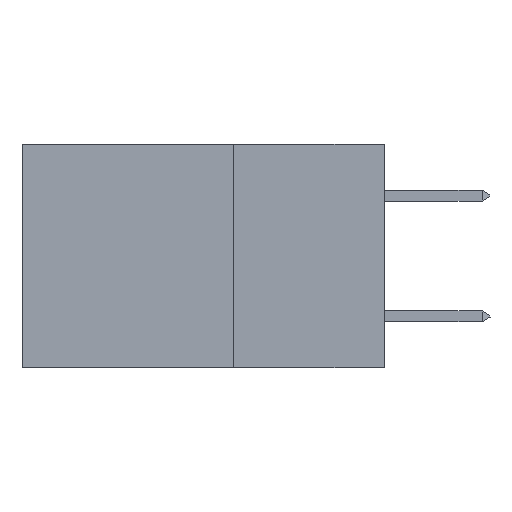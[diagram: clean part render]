
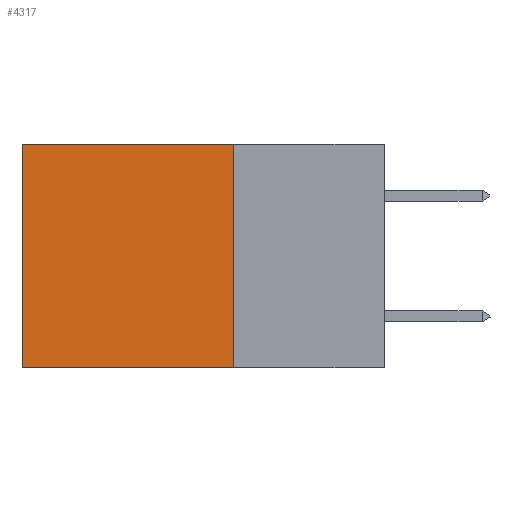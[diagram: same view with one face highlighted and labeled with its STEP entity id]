
A CAD part, left-side view. The second image highlights one B-rep face of the part: STEP entity #4317.
In plain terms, the highlighted planar face has unit normal (-1, 0, 0).
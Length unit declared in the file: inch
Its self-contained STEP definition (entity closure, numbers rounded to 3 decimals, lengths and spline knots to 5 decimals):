
#6 = CARTESIAN_POINT ( 'NONE',  ( 0.2875, 0.25, -0.37 ) ) ;
#36 = ORIENTED_EDGE ( 'NONE', *, *, #13482, .F. ) ;
#254 = ORIENTED_EDGE ( 'NONE', *, *, #1266, .T. ) ;
#265 = EDGE_CURVE ( 'NONE', #1464, #14253, #1152, .T. ) ;
#725 = DIRECTION ( 'NONE',  ( 0., 1., 0. ) ) ;
#787 = VECTOR ( 'NONE', #8856, 39.37008 ) ;
#1096 = DIRECTION ( 'NONE',  ( 0., 1., 0. ) ) ;
#1152 = LINE ( 'NONE', #13448, #787 ) ;
#1266 = EDGE_CURVE ( 'NONE', #7739, #12143, #2345, .T. ) ;
#1464 = VERTEX_POINT ( 'NONE', #4417 ) ;
#1869 = CARTESIAN_POINT ( 'NONE',  ( 0.2875, 0.25, -0.37 ) ) ;
#2345 = LINE ( 'NONE', #13073, #2856 ) ;
#2378 = DIRECTION ( 'NONE',  ( 1., 0., 0. ) ) ;
#2856 = VECTOR ( 'NONE', #13174, 39.37008 ) ;
#2892 = EDGE_CURVE ( 'NONE', #1464, #7739, #4488, .T. ) ;
#3500 = LINE ( 'NONE', #1869, #11552 ) ;
#4007 = ORIENTED_EDGE ( 'NONE', *, *, #2892, .T. ) ;
#4317 = ADVANCED_FACE ( 'NONE', ( #4813 ), #6948, .F. ) ;
#4417 = CARTESIAN_POINT ( 'NONE',  ( 0.2875, 0.25, 0. ) ) ;
#4488 = LINE ( 'NONE', #6894, #11859 ) ;
#4813 = FACE_OUTER_BOUND ( 'NONE', #9438, .T. ) ;
#5140 = ORIENTED_EDGE ( 'NONE', *, *, #265, .F. ) ;
#6894 = CARTESIAN_POINT ( 'NONE',  ( 0.2875, 0.25, 0. ) ) ;
#6948 = PLANE ( 'NONE',  #14022 ) ;
#7739 = VERTEX_POINT ( 'NONE', #14398 ) ;
#8856 = DIRECTION ( 'NONE',  ( 0., 0., -1. ) ) ;
#9026 = CARTESIAN_POINT ( 'NONE',  ( 0.2875, 0.6, -0.37 ) ) ;
#9196 = CARTESIAN_POINT ( 'NONE',  ( 0.2875, 0.25, 0. ) ) ;
#9438 = EDGE_LOOP ( 'NONE', ( #254, #36, #5140, #4007 ) ) ;
#10353 = DIRECTION ( 'NONE',  ( 0., 0., -1. ) ) ;
#11552 = VECTOR ( 'NONE', #725, 39.37008 ) ;
#11859 = VECTOR ( 'NONE', #1096, 39.37008 ) ;
#12143 = VERTEX_POINT ( 'NONE', #9026 ) ;
#13073 = CARTESIAN_POINT ( 'NONE',  ( 0.2875, 0.6, 0. ) ) ;
#13174 = DIRECTION ( 'NONE',  ( 0., 0., -1. ) ) ;
#13448 = CARTESIAN_POINT ( 'NONE',  ( 0.2875, 0.25, 0. ) ) ;
#13482 = EDGE_CURVE ( 'NONE', #14253, #12143, #3500, .T. ) ;
#14022 = AXIS2_PLACEMENT_3D ( 'NONE', #9196, #2378, #10353 ) ;
#14253 = VERTEX_POINT ( 'NONE', #6 ) ;
#14398 = CARTESIAN_POINT ( 'NONE',  ( 0.2875, 0.6, 0. ) ) ;
